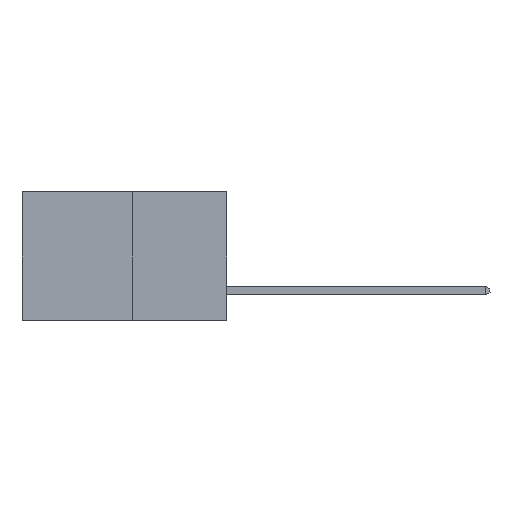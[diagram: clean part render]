
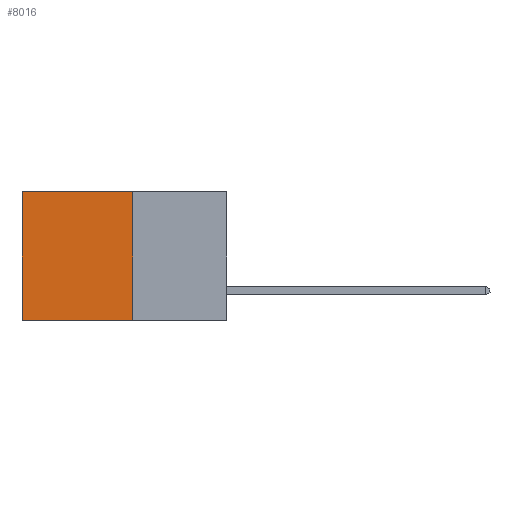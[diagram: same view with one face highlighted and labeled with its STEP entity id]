
A CAD part, left-side view. The second image highlights one B-rep face of the part: STEP entity #8016.
In plain terms, the highlighted planar face has unit normal (-1, 0, 0).
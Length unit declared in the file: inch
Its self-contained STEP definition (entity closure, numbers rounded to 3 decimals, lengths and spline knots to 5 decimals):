
#42 = PLANE ( 'NONE',  #7591 ) ;
#167 = DIRECTION ( 'NONE',  ( 0., 0., -1. ) ) ;
#182 = DIRECTION ( 'NONE',  ( 1., 0., 0. ) ) ;
#413 = VECTOR ( 'NONE', #6339, 39.37008 ) ;
#495 = CARTESIAN_POINT ( 'NONE',  ( 0.277, 0.27, -0.37 ) ) ;
#789 = VERTEX_POINT ( 'NONE', #1112 ) ;
#1024 = VERTEX_POINT ( 'NONE', #7681 ) ;
#1112 = CARTESIAN_POINT ( 'NONE',  ( 0.277, 0.59, 0. ) ) ;
#1271 = CARTESIAN_POINT ( 'NONE',  ( 0.277, 0.59, -0.37 ) ) ;
#1287 = CARTESIAN_POINT ( 'NONE',  ( 0.277, 0.27, 0. ) ) ;
#1492 = DIRECTION ( 'NONE',  ( 0., 1., 0. ) ) ;
#2455 = VECTOR ( 'NONE', #1492, 39.37008 ) ;
#2594 = CARTESIAN_POINT ( 'NONE',  ( 0.277, 0.27, -0.37 ) ) ;
#3256 = EDGE_CURVE ( 'NONE', #1024, #7643, #7467, .T. ) ;
#3721 = DIRECTION ( 'NONE',  ( 0., 0., -1. ) ) ;
#3866 = VERTEX_POINT ( 'NONE', #1287 ) ;
#4160 = EDGE_CURVE ( 'NONE', #3866, #1024, #5595, .T. ) ;
#4463 = LINE ( 'NONE', #7624, #2455 ) ;
#5331 = EDGE_CURVE ( 'NONE', #3866, #789, #4463, .T. ) ;
#5595 = LINE ( 'NONE', #2594, #7216 ) ;
#5835 = VECTOR ( 'NONE', #8017, 39.37008 ) ;
#5997 = LINE ( 'NONE', #1271, #413 ) ;
#6062 = ORIENTED_EDGE ( 'NONE', *, *, #4160, .F. ) ;
#6339 = DIRECTION ( 'NONE',  ( 0., 0., -1. ) ) ;
#6362 = EDGE_LOOP ( 'NONE', ( #8730, #6495, #6062, #7882 ) ) ;
#6495 = ORIENTED_EDGE ( 'NONE', *, *, #3256, .F. ) ;
#6583 = FACE_OUTER_BOUND ( 'NONE', #6362, .T. ) ;
#6793 = EDGE_CURVE ( 'NONE', #789, #7643, #5997, .T. ) ;
#7019 = CARTESIAN_POINT ( 'NONE',  ( 0.277, 0.27, -0.37 ) ) ;
#7216 = VECTOR ( 'NONE', #3721, 39.37008 ) ;
#7467 = LINE ( 'NONE', #7019, #5835 ) ;
#7591 = AXIS2_PLACEMENT_3D ( 'NONE', #495, #182, #167 ) ;
#7624 = CARTESIAN_POINT ( 'NONE',  ( 0.277, 0.27, 0. ) ) ;
#7643 = VERTEX_POINT ( 'NONE', #9420 ) ;
#7681 = CARTESIAN_POINT ( 'NONE',  ( 0.277, 0.27, -0.37 ) ) ;
#7882 = ORIENTED_EDGE ( 'NONE', *, *, #5331, .T. ) ;
#8016 = ADVANCED_FACE ( 'NONE', ( #6583 ), #42, .F. ) ;
#8017 = DIRECTION ( 'NONE',  ( 0., 1., 0. ) ) ;
#8730 = ORIENTED_EDGE ( 'NONE', *, *, #6793, .T. ) ;
#9420 = CARTESIAN_POINT ( 'NONE',  ( 0.277, 0.59, -0.37 ) ) ;
